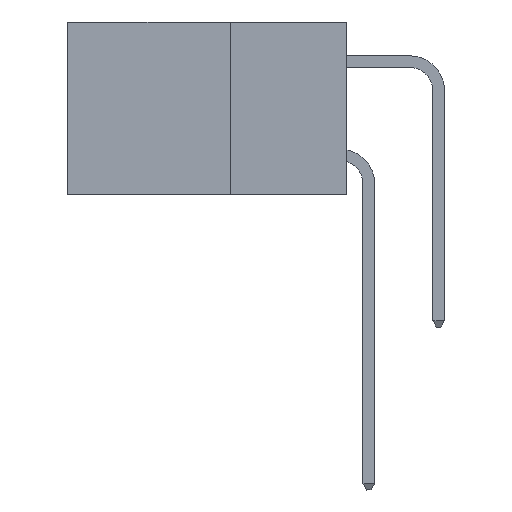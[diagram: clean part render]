
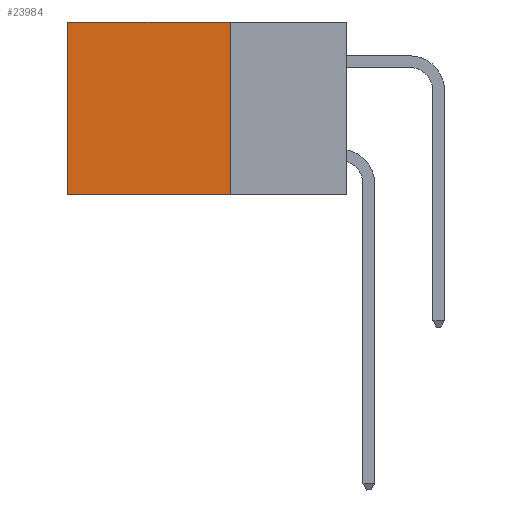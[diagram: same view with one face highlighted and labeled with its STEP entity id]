
A CAD part, left-side view. The second image highlights one B-rep face of the part: STEP entity #23984.
In plain terms, the highlighted planar face has unit normal (-1, 0, 0).
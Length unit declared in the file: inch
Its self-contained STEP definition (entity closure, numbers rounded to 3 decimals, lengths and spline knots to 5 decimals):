
#325 = DIRECTION ( 'NONE',  ( 0., 0., -1. ) ) ;
#556 = ORIENTED_EDGE ( 'NONE', *, *, #6851, .T. ) ;
#616 = CARTESIAN_POINT ( 'NONE',  ( 0.2875, 0.25, 0. ) ) ;
#2682 = EDGE_CURVE ( 'NONE', #10274, #11556, #12231, .T. ) ;
#4483 = CARTESIAN_POINT ( 'NONE',  ( 0.2875, 0.25, 0. ) ) ;
#5129 = VECTOR ( 'NONE', #325, 39.37008 ) ;
#5190 = CARTESIAN_POINT ( 'NONE',  ( 0.2875, 0.6, -0.37 ) ) ;
#5302 = VECTOR ( 'NONE', #24429, 39.37008 ) ;
#5710 = DIRECTION ( 'NONE',  ( 0., 0., -1. ) ) ;
#5996 = LINE ( 'NONE', #22362, #7781 ) ;
#6851 = EDGE_CURVE ( 'NONE', #10274, #30151, #29808, .T. ) ;
#7431 = CARTESIAN_POINT ( 'NONE',  ( 0.2875, 0.6, 0. ) ) ;
#7781 = VECTOR ( 'NONE', #5710, 39.37008 ) ;
#9327 = VERTEX_POINT ( 'NONE', #5190 ) ;
#9336 = CARTESIAN_POINT ( 'NONE',  ( 0.2875, 0.25, 0. ) ) ;
#9904 = CARTESIAN_POINT ( 'NONE',  ( 0.2875, 0.25, -0.37 ) ) ;
#10092 = PLANE ( 'NONE',  #22434 ) ;
#10274 = VERTEX_POINT ( 'NONE', #9336 ) ;
#10832 = EDGE_CURVE ( 'NONE', #11556, #9327, #28895, .T. ) ;
#11556 = VERTEX_POINT ( 'NONE', #23595 ) ;
#12134 = DIRECTION ( 'NONE',  ( 1., 0., 0. ) ) ;
#12231 = LINE ( 'NONE', #616, #5129 ) ;
#12265 = DIRECTION ( 'NONE',  ( 0., 0., -1. ) ) ;
#17141 = EDGE_LOOP ( 'NONE', ( #26601, #20668, #25437, #556 ) ) ;
#20668 = ORIENTED_EDGE ( 'NONE', *, *, #10832, .F. ) ;
#22362 = CARTESIAN_POINT ( 'NONE',  ( 0.2875, 0.6, 0. ) ) ;
#22434 = AXIS2_PLACEMENT_3D ( 'NONE', #28609, #12134, #12265 ) ;
#23595 = CARTESIAN_POINT ( 'NONE',  ( 0.2875, 0.25, -0.37 ) ) ;
#23984 = ADVANCED_FACE ( 'NONE', ( #24287 ), #10092, .F. ) ;
#24287 = FACE_OUTER_BOUND ( 'NONE', #17141, .T. ) ;
#24429 = DIRECTION ( 'NONE',  ( 0., 1., 0. ) ) ;
#25437 = ORIENTED_EDGE ( 'NONE', *, *, #2682, .F. ) ;
#25472 = DIRECTION ( 'NONE',  ( 0., 1., 0. ) ) ;
#26439 = EDGE_CURVE ( 'NONE', #30151, #9327, #5996, .T. ) ;
#26601 = ORIENTED_EDGE ( 'NONE', *, *, #26439, .T. ) ;
#28609 = CARTESIAN_POINT ( 'NONE',  ( 0.2875, 0.25, 0. ) ) ;
#28895 = LINE ( 'NONE', #9904, #5302 ) ;
#29808 = LINE ( 'NONE', #4483, #30360 ) ;
#30151 = VERTEX_POINT ( 'NONE', #7431 ) ;
#30360 = VECTOR ( 'NONE', #25472, 39.37008 ) ;
